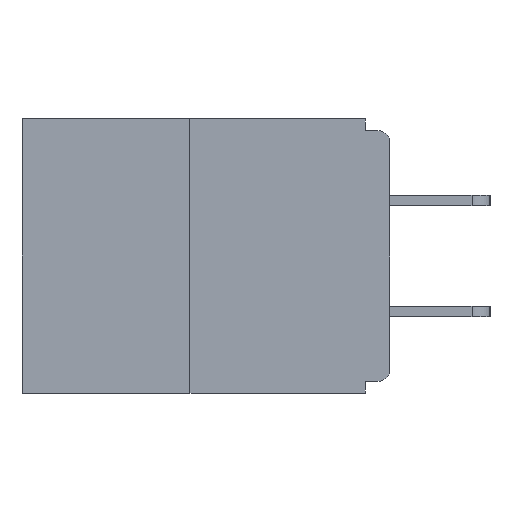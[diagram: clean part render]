
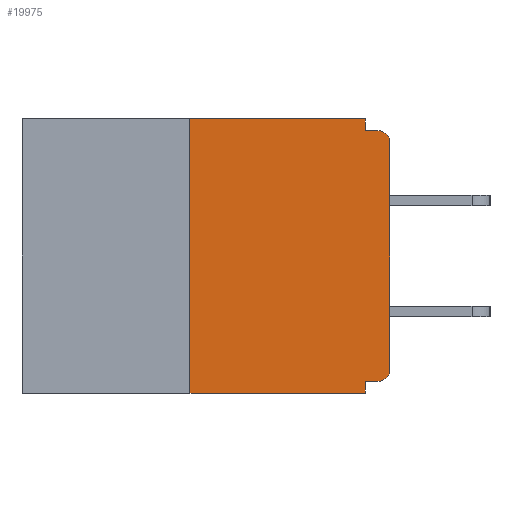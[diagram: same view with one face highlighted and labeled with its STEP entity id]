
A CAD part, left-side view. The second image highlights one B-rep face of the part: STEP entity #19975.
In plain terms, the highlighted planar face has unit normal (-1, 0, 0).
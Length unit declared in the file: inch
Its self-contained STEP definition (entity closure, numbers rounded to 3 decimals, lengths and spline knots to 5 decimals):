
#610 = ORIENTED_EDGE ( 'NONE', *, *, #9263, .F. ) ;
#1402 = VERTEX_POINT ( 'NONE', #17790 ) ;
#1468 = CARTESIAN_POINT ( 'NONE',  ( 0., 0.25, 0. ) ) ;
#1708 = CARTESIAN_POINT ( 'NONE',  ( 0., 0., -0.03 ) ) ;
#1855 = CIRCLE ( 'NONE', #7221, 0.015 ) ;
#1973 = VERTEX_POINT ( 'NONE', #12166 ) ;
#2030 = VERTEX_POINT ( 'NONE', #12520 ) ;
#2274 = LINE ( 'NONE', #13510, #11607 ) ;
#2453 = DIRECTION ( 'NONE',  ( 0., 0., 1. ) ) ;
#2960 = CARTESIAN_POINT ( 'NONE',  ( 0., 0.46, 0. ) ) ;
#3012 = CARTESIAN_POINT ( 'NONE',  ( 0., 0.031, -0.343 ) ) ;
#3311 = DIRECTION ( 'NONE',  ( 0., -1., 0. ) ) ;
#3324 = ORIENTED_EDGE ( 'NONE', *, *, #11326, .F. ) ;
#3385 = AXIS2_PLACEMENT_3D ( 'NONE', #13471, #7483, #13537 ) ;
#4048 = EDGE_CURVE ( 'NONE', #13521, #14567, #4926, .T. ) ;
#4655 = LINE ( 'NONE', #3012, #18157 ) ;
#4926 = LINE ( 'NONE', #13228, #13525 ) ;
#5233 = VECTOR ( 'NONE', #12656, 39.37008 ) ;
#5254 = ORIENTED_EDGE ( 'NONE', *, *, #4048, .F. ) ;
#5275 = DIRECTION ( 'NONE',  ( 0., 1., 0. ) ) ;
#5325 = CARTESIAN_POINT ( 'NONE',  ( 0., 0.25, 0. ) ) ;
#5760 = EDGE_CURVE ( 'NONE', #14704, #8193, #17151, .T. ) ;
#5867 = VECTOR ( 'NONE', #12404, 39.37008 ) ;
#5942 = CARTESIAN_POINT ( 'NONE',  ( 0., 0.46, -0.343 ) ) ;
#5987 = VECTOR ( 'NONE', #3311, 39.37008 ) ;
#6251 = CARTESIAN_POINT ( 'NONE',  ( 0., 0.46, 0. ) ) ;
#6282 = EDGE_CURVE ( 'NONE', #8193, #8313, #8563, .T. ) ;
#6398 = ORIENTED_EDGE ( 'NONE', *, *, #9178, .T. ) ;
#6402 = CARTESIAN_POINT ( 'NONE',  ( 0., 0.031, -0.343 ) ) ;
#6567 = CARTESIAN_POINT ( 'NONE',  ( 0., 0.031, 0. ) ) ;
#6965 = LINE ( 'NONE', #7842, #5987 ) ;
#7221 = AXIS2_PLACEMENT_3D ( 'NONE', #18002, #17925, #14971 ) ;
#7414 = EDGE_LOOP ( 'NONE', ( #8811, #19308, #6398, #3324, #5254, #16072, #15091, #8368, #17366, #610 ) ) ;
#7483 = DIRECTION ( 'NONE',  ( -1., 0., 0. ) ) ;
#7762 = PLANE ( 'NONE',  #8495 ) ;
#7842 = CARTESIAN_POINT ( 'NONE',  ( 0., 0., -0.015 ) ) ;
#8193 = VERTEX_POINT ( 'NONE', #5325 ) ;
#8249 = VERTEX_POINT ( 'NONE', #1708 ) ;
#8300 = CARTESIAN_POINT ( 'NONE',  ( 0., 0.031, -0.328 ) ) ;
#8313 = VERTEX_POINT ( 'NONE', #6567 ) ;
#8368 = ORIENTED_EDGE ( 'NONE', *, *, #10641, .T. ) ;
#8391 = CARTESIAN_POINT ( 'NONE',  ( 0., 0.015, -0.328 ) ) ;
#8495 = AXIS2_PLACEMENT_3D ( 'NONE', #6251, #13869, #14135 ) ;
#8563 = LINE ( 'NONE', #2960, #11258 ) ;
#8811 = ORIENTED_EDGE ( 'NONE', *, *, #6282, .F. ) ;
#9178 = EDGE_CURVE ( 'NONE', #14704, #13332, #16028, .T. ) ;
#9263 = EDGE_CURVE ( 'NONE', #8313, #1402, #19467, .T. ) ;
#10641 = EDGE_CURVE ( 'NONE', #8249, #2030, #11560, .T. ) ;
#10936 = DIRECTION ( 'NONE',  ( 0., 0., -1. ) ) ;
#11206 = FACE_OUTER_BOUND ( 'NONE', #7414, .T. ) ;
#11258 = VECTOR ( 'NONE', #11867, 39.37008 ) ;
#11326 = EDGE_CURVE ( 'NONE', #14567, #13332, #4655, .T. ) ;
#11560 = CIRCLE ( 'NONE', #3385, 0.015 ) ;
#11607 = VECTOR ( 'NONE', #2453, 39.37008 ) ;
#11867 = DIRECTION ( 'NONE',  ( 0., -1., 0. ) ) ;
#12166 = CARTESIAN_POINT ( 'NONE',  ( 0., 0., -0.313 ) ) ;
#12404 = DIRECTION ( 'NONE',  ( 0., 0., 1. ) ) ;
#12520 = CARTESIAN_POINT ( 'NONE',  ( 0., 0.015, -0.015 ) ) ;
#12656 = DIRECTION ( 'NONE',  ( 0., 0., -1. ) ) ;
#13228 = CARTESIAN_POINT ( 'NONE',  ( 0., 0., -0.328 ) ) ;
#13332 = VERTEX_POINT ( 'NONE', #6402 ) ;
#13471 = CARTESIAN_POINT ( 'NONE',  ( 0., 0.015, -0.03 ) ) ;
#13510 = CARTESIAN_POINT ( 'NONE',  ( 0., 0., 0. ) ) ;
#13521 = VERTEX_POINT ( 'NONE', #8391 ) ;
#13525 = VECTOR ( 'NONE', #5275, 39.37008 ) ;
#13537 = DIRECTION ( 'NONE',  ( 0., 0., -1. ) ) ;
#13640 = EDGE_CURVE ( 'NONE', #13521, #1973, #1855, .T. ) ;
#13869 = DIRECTION ( 'NONE',  ( 1., 0., 0. ) ) ;
#14135 = DIRECTION ( 'NONE',  ( 0., 0., -1. ) ) ;
#14567 = VERTEX_POINT ( 'NONE', #8300 ) ;
#14704 = VERTEX_POINT ( 'NONE', #17068 ) ;
#14971 = DIRECTION ( 'NONE',  ( 0., 0., -1. ) ) ;
#15091 = ORIENTED_EDGE ( 'NONE', *, *, #15772, .T. ) ;
#15337 = EDGE_CURVE ( 'NONE', #1402, #2030, #6965, .T. ) ;
#15346 = DIRECTION ( 'NONE',  ( 0., -1., 0. ) ) ;
#15772 = EDGE_CURVE ( 'NONE', #1973, #8249, #2274, .T. ) ;
#16028 = LINE ( 'NONE', #5942, #16271 ) ;
#16072 = ORIENTED_EDGE ( 'NONE', *, *, #13640, .T. ) ;
#16271 = VECTOR ( 'NONE', #15346, 39.37008 ) ;
#17068 = CARTESIAN_POINT ( 'NONE',  ( 0., 0.25, -0.343 ) ) ;
#17151 = LINE ( 'NONE', #1468, #5867 ) ;
#17366 = ORIENTED_EDGE ( 'NONE', *, *, #15337, .F. ) ;
#17790 = CARTESIAN_POINT ( 'NONE',  ( 0., 0.031, -0.015 ) ) ;
#17925 = DIRECTION ( 'NONE',  ( -1., 0., 0. ) ) ;
#18002 = CARTESIAN_POINT ( 'NONE',  ( 0., 0.015, -0.313 ) ) ;
#18157 = VECTOR ( 'NONE', #10936, 39.37008 ) ;
#19308 = ORIENTED_EDGE ( 'NONE', *, *, #5760, .F. ) ;
#19467 = LINE ( 'NONE', #20302, #5233 ) ;
#19975 = ADVANCED_FACE ( 'NONE', ( #11206 ), #7762, .F. ) ;
#20302 = CARTESIAN_POINT ( 'NONE',  ( 0., 0.031, 0. ) ) ;
